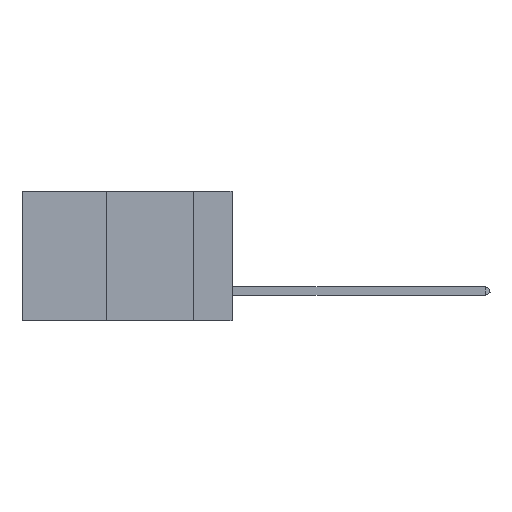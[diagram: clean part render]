
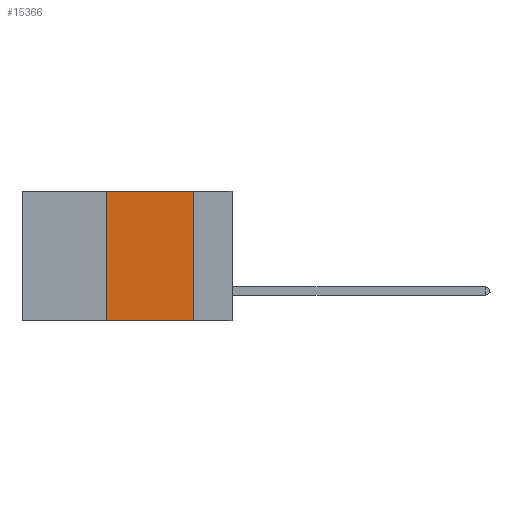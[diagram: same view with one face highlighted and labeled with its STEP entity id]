
A CAD part, left-side view. The second image highlights one B-rep face of the part: STEP entity #15366.
In plain terms, the highlighted planar face has unit normal (-1, 0, 0).
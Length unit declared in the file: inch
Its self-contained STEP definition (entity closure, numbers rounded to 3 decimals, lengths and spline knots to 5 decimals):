
#126 = AXIS2_PLACEMENT_3D ( 'NONE', #4027, #21960, #16449 ) ;
#818 = ORIENTED_EDGE ( 'NONE', *, *, #13959, .F. ) ;
#1235 = EDGE_CURVE ( 'NONE', #19320, #4556, #22123, .T. ) ;
#1447 = VERTEX_POINT ( 'NONE', #10600 ) ;
#2263 = DIRECTION ( 'NONE',  ( 0., -1., 0. ) ) ;
#2447 = PLANE ( 'NONE',  #126 ) ;
#2518 = ORIENTED_EDGE ( 'NONE', *, *, #5645, .F. ) ;
#2998 = CARTESIAN_POINT ( 'NONE',  ( 0., 0.6, 0. ) ) ;
#4027 = CARTESIAN_POINT ( 'NONE',  ( 0., 0.6, 0. ) ) ;
#4233 = ORIENTED_EDGE ( 'NONE', *, *, #18478, .T. ) ;
#4556 = VERTEX_POINT ( 'NONE', #4717 ) ;
#4717 = CARTESIAN_POINT ( 'NONE',  ( 0., 0.36, 0. ) ) ;
#4788 = CARTESIAN_POINT ( 'NONE',  ( 0., 0.36, 0. ) ) ;
#5271 = LINE ( 'NONE', #11202, #12787 ) ;
#5435 = EDGE_LOOP ( 'NONE', ( #818, #2518, #10623, #4233 ) ) ;
#5645 = EDGE_CURVE ( 'NONE', #4556, #1447, #15386, .T. ) ;
#7271 = DIRECTION ( 'NONE',  ( 0., 0., -1. ) ) ;
#10600 = CARTESIAN_POINT ( 'NONE',  ( 0., 0.11, 0. ) ) ;
#10623 = ORIENTED_EDGE ( 'NONE', *, *, #1235, .F. ) ;
#11202 = CARTESIAN_POINT ( 'NONE',  ( 0., 0.6, -0.37 ) ) ;
#12787 = VECTOR ( 'NONE', #2263, 39.37008 ) ;
#13582 = DIRECTION ( 'NONE',  ( 0., -1., 0. ) ) ;
#13959 = EDGE_CURVE ( 'NONE', #1447, #17860, #16309, .T. ) ;
#14342 = CARTESIAN_POINT ( 'NONE',  ( 0., 0.11, 0. ) ) ;
#14581 = VECTOR ( 'NONE', #13582, 39.37008 ) ;
#15366 = ADVANCED_FACE ( 'NONE', ( #20944 ), #2447, .F. ) ;
#15386 = LINE ( 'NONE', #2998, #14581 ) ;
#16309 = LINE ( 'NONE', #14342, #21028 ) ;
#16449 = DIRECTION ( 'NONE',  ( 0., 0., -1. ) ) ;
#17388 = DIRECTION ( 'NONE',  ( 0., 0., 1. ) ) ;
#17860 = VERTEX_POINT ( 'NONE', #19439 ) ;
#18478 = EDGE_CURVE ( 'NONE', #19320, #17860, #5271, .T. ) ;
#19320 = VERTEX_POINT ( 'NONE', #21119 ) ;
#19439 = CARTESIAN_POINT ( 'NONE',  ( 0., 0.11, -0.37 ) ) ;
#20428 = VECTOR ( 'NONE', #17388, 39.37008 ) ;
#20944 = FACE_OUTER_BOUND ( 'NONE', #5435, .T. ) ;
#21028 = VECTOR ( 'NONE', #7271, 39.37008 ) ;
#21119 = CARTESIAN_POINT ( 'NONE',  ( 0., 0.36, -0.37 ) ) ;
#21960 = DIRECTION ( 'NONE',  ( 1., 0., 0. ) ) ;
#22123 = LINE ( 'NONE', #4788, #20428 ) ;
